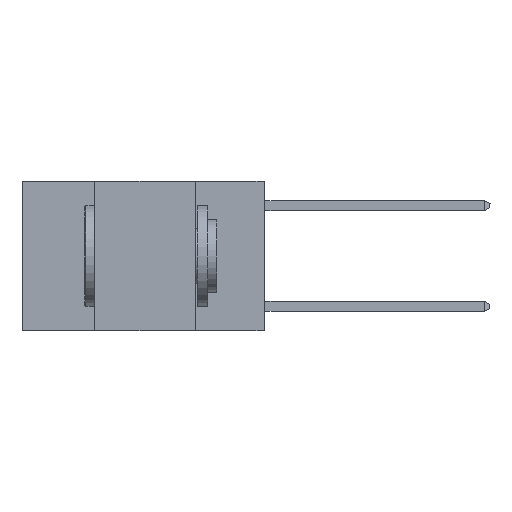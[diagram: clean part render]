
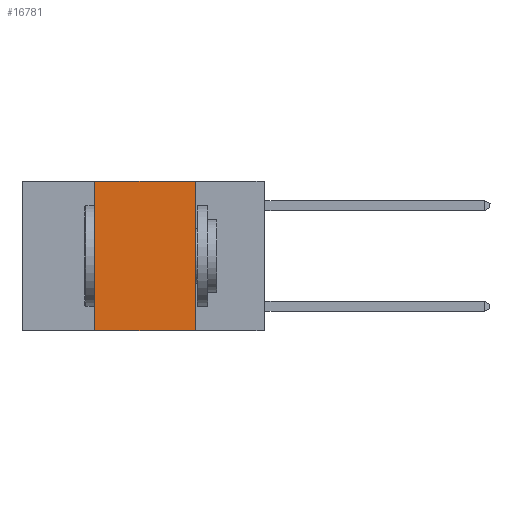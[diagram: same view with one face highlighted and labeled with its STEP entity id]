
A CAD part, left-side view. The second image highlights one B-rep face of the part: STEP entity #16781.
In plain terms, the highlighted planar face has unit normal (-1, 0, 0).
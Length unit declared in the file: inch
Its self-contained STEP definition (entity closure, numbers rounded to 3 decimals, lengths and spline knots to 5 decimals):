
#1192 = LINE ( 'NONE', #1911, #7945 ) ;
#1666 = VERTEX_POINT ( 'NONE', #10799 ) ;
#1911 = CARTESIAN_POINT ( 'NONE',  ( 0., 0.17, 0. ) ) ;
#2347 = CARTESIAN_POINT ( 'NONE',  ( 0., 0.6, 0. ) ) ;
#3153 = CARTESIAN_POINT ( 'NONE',  ( 0., 0.17, -0.37 ) ) ;
#3707 = DIRECTION ( 'NONE',  ( 0., 0., -1. ) ) ;
#4068 = EDGE_CURVE ( 'NONE', #1666, #6835, #6590, .T. ) ;
#4705 = DIRECTION ( 'NONE',  ( 0., -1., 0. ) ) ;
#4869 = FACE_OUTER_BOUND ( 'NONE', #7439, .T. ) ;
#5056 = VECTOR ( 'NONE', #4705, 39.37008 ) ;
#5274 = DIRECTION ( 'NONE',  ( 0., -1., 0. ) ) ;
#5505 = LINE ( 'NONE', #7368, #5056 ) ;
#6384 = ORIENTED_EDGE ( 'NONE', *, *, #12279, .F. ) ;
#6590 = LINE ( 'NONE', #7803, #17201 ) ;
#6835 = VERTEX_POINT ( 'NONE', #8570 ) ;
#7215 = ORIENTED_EDGE ( 'NONE', *, *, #4068, .F. ) ;
#7368 = CARTESIAN_POINT ( 'NONE',  ( 0., 0.6, 0. ) ) ;
#7439 = EDGE_LOOP ( 'NONE', ( #6384, #15119, #7215, #8484 ) ) ;
#7803 = CARTESIAN_POINT ( 'NONE',  ( 0., 0.42, 0. ) ) ;
#7945 = VECTOR ( 'NONE', #16663, 39.37008 ) ;
#8484 = ORIENTED_EDGE ( 'NONE', *, *, #17344, .T. ) ;
#8570 = CARTESIAN_POINT ( 'NONE',  ( 0., 0.42, 0. ) ) ;
#8689 = CARTESIAN_POINT ( 'NONE',  ( 0., 0.17, 0. ) ) ;
#9158 = DIRECTION ( 'NONE',  ( 0., 0., 1. ) ) ;
#9490 = LINE ( 'NONE', #15936, #13033 ) ;
#10196 = EDGE_CURVE ( 'NONE', #6835, #12292, #5505, .T. ) ;
#10419 = PLANE ( 'NONE',  #16700 ) ;
#10799 = CARTESIAN_POINT ( 'NONE',  ( 0., 0.42, -0.37 ) ) ;
#11742 = DIRECTION ( 'NONE',  ( 1., 0., 0. ) ) ;
#12279 = EDGE_CURVE ( 'NONE', #12292, #13938, #1192, .T. ) ;
#12292 = VERTEX_POINT ( 'NONE', #8689 ) ;
#13033 = VECTOR ( 'NONE', #5274, 39.37008 ) ;
#13938 = VERTEX_POINT ( 'NONE', #3153 ) ;
#15119 = ORIENTED_EDGE ( 'NONE', *, *, #10196, .F. ) ;
#15936 = CARTESIAN_POINT ( 'NONE',  ( 0., 0.6, -0.37 ) ) ;
#16663 = DIRECTION ( 'NONE',  ( 0., 0., -1. ) ) ;
#16700 = AXIS2_PLACEMENT_3D ( 'NONE', #2347, #11742, #3707 ) ;
#16781 = ADVANCED_FACE ( 'NONE', ( #4869 ), #10419, .F. ) ;
#17201 = VECTOR ( 'NONE', #9158, 39.37008 ) ;
#17344 = EDGE_CURVE ( 'NONE', #1666, #13938, #9490, .T. ) ;
